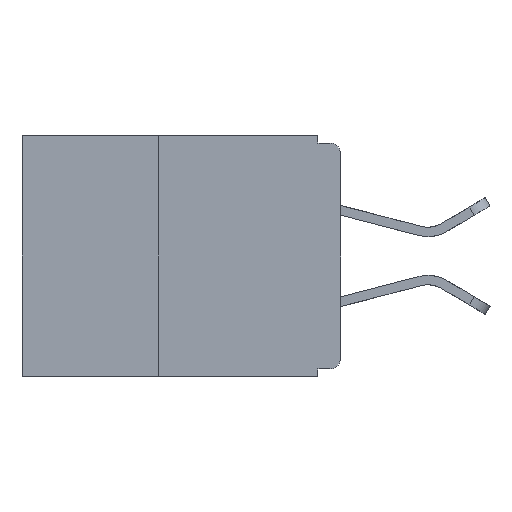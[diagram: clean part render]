
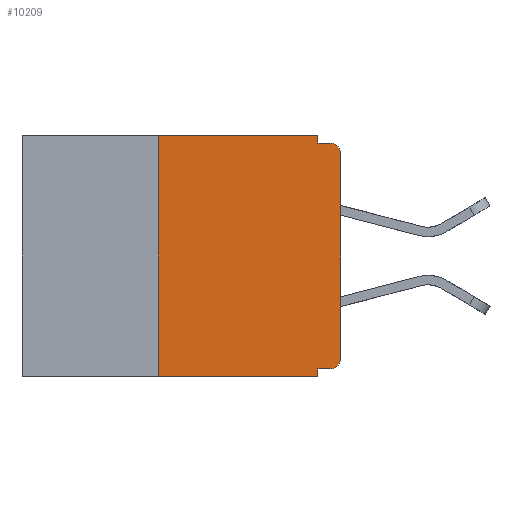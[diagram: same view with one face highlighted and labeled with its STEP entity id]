
A CAD part, left-side view. The second image highlights one B-rep face of the part: STEP entity #10209.
In plain terms, the highlighted planar face has unit normal (-1, 0, 0).
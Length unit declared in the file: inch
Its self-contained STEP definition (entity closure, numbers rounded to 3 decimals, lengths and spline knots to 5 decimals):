
#636 = EDGE_CURVE ( 'NONE', #15455, #7321, #12618, .T. ) ;
#751 = ORIENTED_EDGE ( 'NONE', *, *, #3213, .T. ) ;
#898 = ORIENTED_EDGE ( 'NONE', *, *, #8233, .F. ) ;
#1007 = DIRECTION ( 'NONE',  ( 0., 0., -1. ) ) ;
#1557 = CARTESIAN_POINT ( 'NONE',  ( 0., 0.25, -0.33 ) ) ;
#1671 = VECTOR ( 'NONE', #1989, 39.37008 ) ;
#1704 = CIRCLE ( 'NONE', #5089, 0.015 ) ;
#1886 = CARTESIAN_POINT ( 'NONE',  ( 0., 0., -0.305 ) ) ;
#1941 = DIRECTION ( 'NONE',  ( 0., 0., 1. ) ) ;
#1989 = DIRECTION ( 'NONE',  ( 0., 0., -1. ) ) ;
#2018 = EDGE_CURVE ( 'NONE', #2727, #15455, #16123, .T. ) ;
#2071 = CARTESIAN_POINT ( 'NONE',  ( 0., 0.031, -0.33 ) ) ;
#2339 = EDGE_CURVE ( 'NONE', #16209, #7997, #4361, .T. ) ;
#2345 = VERTEX_POINT ( 'NONE', #9703 ) ;
#2727 = VERTEX_POINT ( 'NONE', #14366 ) ;
#3054 = VECTOR ( 'NONE', #15130, 39.37008 ) ;
#3213 = EDGE_CURVE ( 'NONE', #2345, #16504, #1704, .T. ) ;
#3685 = DIRECTION ( 'NONE',  ( 0., 1., 0. ) ) ;
#3760 = CARTESIAN_POINT ( 'NONE',  ( 0., 0., -0.32 ) ) ;
#3947 = CARTESIAN_POINT ( 'NONE',  ( 0., 0.031, 0. ) ) ;
#4096 = EDGE_CURVE ( 'NONE', #11696, #5574, #15088, .T. ) ;
#4169 = VECTOR ( 'NONE', #15576, 39.37008 ) ;
#4361 = CIRCLE ( 'NONE', #6945, 0.015 ) ;
#4493 = ORIENTED_EDGE ( 'NONE', *, *, #15835, .F. ) ;
#4729 = DIRECTION ( 'NONE',  ( 0., 0., -1. ) ) ;
#4941 = LINE ( 'NONE', #10055, #8869 ) ;
#5088 = CARTESIAN_POINT ( 'NONE',  ( 0., 0.031, -0.01 ) ) ;
#5089 = AXIS2_PLACEMENT_3D ( 'NONE', #14395, #14311, #8387 ) ;
#5170 = ORIENTED_EDGE ( 'NONE', *, *, #636, .F. ) ;
#5198 = CARTESIAN_POINT ( 'NONE',  ( 0., 0., 0. ) ) ;
#5506 = CARTESIAN_POINT ( 'NONE',  ( 0., 0.015, -0.32 ) ) ;
#5574 = VERTEX_POINT ( 'NONE', #7961 ) ;
#5806 = VECTOR ( 'NONE', #1941, 39.37008 ) ;
#6040 = CARTESIAN_POINT ( 'NONE',  ( 0., 0.437, -0.33 ) ) ;
#6051 = AXIS2_PLACEMENT_3D ( 'NONE', #14019, #8891, #1007 ) ;
#6167 = VECTOR ( 'NONE', #3685, 39.37008 ) ;
#6385 = DIRECTION ( 'NONE',  ( 0., -1., 0. ) ) ;
#6400 = CARTESIAN_POINT ( 'NONE',  ( 0., 0.437, 0. ) ) ;
#6548 = DIRECTION ( 'NONE',  ( 0., 0., -1. ) ) ;
#6945 = AXIS2_PLACEMENT_3D ( 'NONE', #7454, #7342, #6548 ) ;
#7099 = ORIENTED_EDGE ( 'NONE', *, *, #2018, .F. ) ;
#7321 = VERTEX_POINT ( 'NONE', #3947 ) ;
#7342 = DIRECTION ( 'NONE',  ( -1., 0., 0. ) ) ;
#7353 = EDGE_CURVE ( 'NONE', #16209, #11696, #9695, .T. ) ;
#7454 = CARTESIAN_POINT ( 'NONE',  ( 0., 0.015, -0.305 ) ) ;
#7961 = CARTESIAN_POINT ( 'NONE',  ( 0., 0.031, -0.33 ) ) ;
#7997 = VERTEX_POINT ( 'NONE', #1886 ) ;
#8233 = EDGE_CURVE ( 'NONE', #15361, #16504, #10075, .T. ) ;
#8351 = ORIENTED_EDGE ( 'NONE', *, *, #15822, .T. ) ;
#8387 = DIRECTION ( 'NONE',  ( 0., 0., -1. ) ) ;
#8869 = VECTOR ( 'NONE', #4729, 39.37008 ) ;
#8891 = DIRECTION ( 'NONE',  ( 1., 0., 0. ) ) ;
#9624 = ORIENTED_EDGE ( 'NONE', *, *, #13550, .T. ) ;
#9695 = LINE ( 'NONE', #3760, #6167 ) ;
#9703 = CARTESIAN_POINT ( 'NONE',  ( 0., 0., -0.025 ) ) ;
#9707 = LINE ( 'NONE', #6040, #11928 ) ;
#9977 = ORIENTED_EDGE ( 'NONE', *, *, #4096, .F. ) ;
#10055 = CARTESIAN_POINT ( 'NONE',  ( 0., 0.031, 0. ) ) ;
#10075 = LINE ( 'NONE', #13858, #3054 ) ;
#10138 = CARTESIAN_POINT ( 'NONE',  ( 0., 0.015, -0.01 ) ) ;
#10161 = PLANE ( 'NONE',  #6051 ) ;
#10209 = ADVANCED_FACE ( 'NONE', ( #14402 ), #10161, .F. ) ;
#10929 = ORIENTED_EDGE ( 'NONE', *, *, #7353, .F. ) ;
#11696 = VERTEX_POINT ( 'NONE', #15570 ) ;
#11865 = CARTESIAN_POINT ( 'NONE',  ( 0., 0.25, 0. ) ) ;
#11928 = VECTOR ( 'NONE', #16361, 39.37008 ) ;
#12558 = ORIENTED_EDGE ( 'NONE', *, *, #2339, .T. ) ;
#12618 = LINE ( 'NONE', #6400, #15957 ) ;
#13246 = EDGE_LOOP ( 'NONE', ( #9624, #751, #898, #4493, #5170, #7099, #8351, #9977, #10929, #12558 ) ) ;
#13550 = EDGE_CURVE ( 'NONE', #7997, #2345, #14964, .T. ) ;
#13858 = CARTESIAN_POINT ( 'NONE',  ( 0., 0., -0.01 ) ) ;
#14019 = CARTESIAN_POINT ( 'NONE',  ( 0., 0.437, 0. ) ) ;
#14311 = DIRECTION ( 'NONE',  ( -1., 0., 0. ) ) ;
#14366 = CARTESIAN_POINT ( 'NONE',  ( 0., 0.25, -0.33 ) ) ;
#14395 = CARTESIAN_POINT ( 'NONE',  ( 0., 0.015, -0.025 ) ) ;
#14402 = FACE_OUTER_BOUND ( 'NONE', #13246, .T. ) ;
#14964 = LINE ( 'NONE', #5198, #4169 ) ;
#15088 = LINE ( 'NONE', #2071, #1671 ) ;
#15130 = DIRECTION ( 'NONE',  ( 0., -1., 0. ) ) ;
#15361 = VERTEX_POINT ( 'NONE', #5088 ) ;
#15455 = VERTEX_POINT ( 'NONE', #11865 ) ;
#15570 = CARTESIAN_POINT ( 'NONE',  ( 0., 0.031, -0.32 ) ) ;
#15576 = DIRECTION ( 'NONE',  ( 0., 0., 1. ) ) ;
#15822 = EDGE_CURVE ( 'NONE', #2727, #5574, #9707, .T. ) ;
#15835 = EDGE_CURVE ( 'NONE', #7321, #15361, #4941, .T. ) ;
#15957 = VECTOR ( 'NONE', #6385, 39.37008 ) ;
#16123 = LINE ( 'NONE', #1557, #5806 ) ;
#16209 = VERTEX_POINT ( 'NONE', #5506 ) ;
#16361 = DIRECTION ( 'NONE',  ( 0., -1., 0. ) ) ;
#16504 = VERTEX_POINT ( 'NONE', #10138 ) ;
